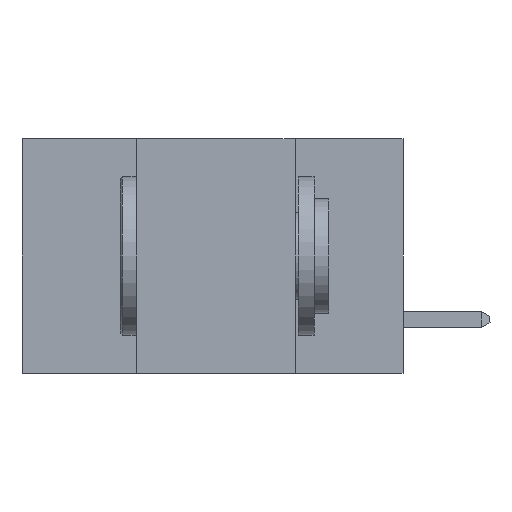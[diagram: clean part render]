
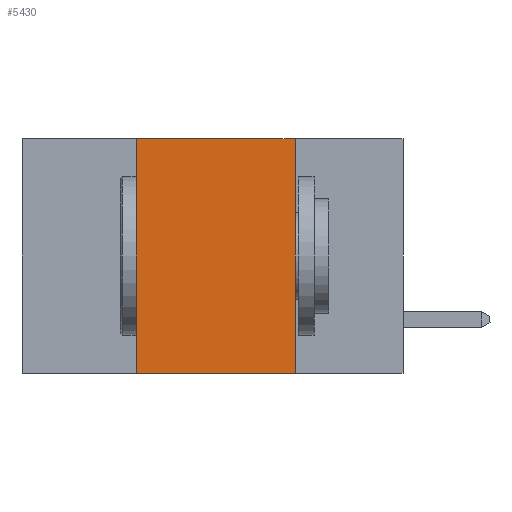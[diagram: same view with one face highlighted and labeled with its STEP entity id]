
A CAD part, left-side view. The second image highlights one B-rep face of the part: STEP entity #5430.
In plain terms, the highlighted planar face has unit normal (-1, 0, 0).
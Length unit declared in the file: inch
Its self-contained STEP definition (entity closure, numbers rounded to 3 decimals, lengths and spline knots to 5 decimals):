
#1590 = VECTOR ( 'NONE', #6048, 39.37008 ) ;
#2099 = VERTEX_POINT ( 'NONE', #13255 ) ;
#2927 = EDGE_LOOP ( 'NONE', ( #19517, #15320, #11067, #22856 ) ) ;
#3734 = CARTESIAN_POINT ( 'NONE',  ( 0., 0.6, 0. ) ) ;
#5430 = ADVANCED_FACE ( 'NONE', ( #18603 ), #16397, .F. ) ;
#5915 = DIRECTION ( 'NONE',  ( 0., 0., -1. ) ) ;
#6048 = DIRECTION ( 'NONE',  ( 0., -1., 0. ) ) ;
#7337 = LINE ( 'NONE', #20715, #1590 ) ;
#8358 = VERTEX_POINT ( 'NONE', #26939 ) ;
#11067 = ORIENTED_EDGE ( 'NONE', *, *, #22249, .F. ) ;
#12402 = CARTESIAN_POINT ( 'NONE',  ( 0., 0.6, 0. ) ) ;
#12452 = VERTEX_POINT ( 'NONE', #20173 ) ;
#13255 = CARTESIAN_POINT ( 'NONE',  ( 0., 0.42, 0. ) ) ;
#15320 = ORIENTED_EDGE ( 'NONE', *, *, #25719, .F. ) ;
#15827 = CARTESIAN_POINT ( 'NONE',  ( 0., 0.17, -0.37 ) ) ;
#15963 = VECTOR ( 'NONE', #16599, 39.37008 ) ;
#16397 = PLANE ( 'NONE',  #23185 ) ;
#16599 = DIRECTION ( 'NONE',  ( 0., -1., 0. ) ) ;
#17939 = CARTESIAN_POINT ( 'NONE',  ( 0., 0.42, 0. ) ) ;
#18466 = DIRECTION ( 'NONE',  ( 1., 0., 0. ) ) ;
#18603 = FACE_OUTER_BOUND ( 'NONE', #2927, .T. ) ;
#19517 = ORIENTED_EDGE ( 'NONE', *, *, #24657, .F. ) ;
#19615 = CARTESIAN_POINT ( 'NONE',  ( 0., 0.17, 0. ) ) ;
#20015 = DIRECTION ( 'NONE',  ( 0., 0., 1. ) ) ;
#20173 = CARTESIAN_POINT ( 'NONE',  ( 0., 0.17, 0. ) ) ;
#20320 = LINE ( 'NONE', #17939, #24641 ) ;
#20570 = VECTOR ( 'NONE', #21779, 39.37008 ) ;
#20715 = CARTESIAN_POINT ( 'NONE',  ( 0., 0.6, -0.37 ) ) ;
#21448 = VERTEX_POINT ( 'NONE', #15827 ) ;
#21779 = DIRECTION ( 'NONE',  ( 0., 0., -1. ) ) ;
#22249 = EDGE_CURVE ( 'NONE', #8358, #2099, #20320, .T. ) ;
#22856 = ORIENTED_EDGE ( 'NONE', *, *, #26970, .T. ) ;
#23185 = AXIS2_PLACEMENT_3D ( 'NONE', #3734, #18466, #5915 ) ;
#24641 = VECTOR ( 'NONE', #20015, 39.37008 ) ;
#24657 = EDGE_CURVE ( 'NONE', #12452, #21448, #26213, .T. ) ;
#25719 = EDGE_CURVE ( 'NONE', #2099, #12452, #27137, .T. ) ;
#26213 = LINE ( 'NONE', #19615, #20570 ) ;
#26939 = CARTESIAN_POINT ( 'NONE',  ( 0., 0.42, -0.37 ) ) ;
#26970 = EDGE_CURVE ( 'NONE', #8358, #21448, #7337, .T. ) ;
#27137 = LINE ( 'NONE', #12402, #15963 ) ;
